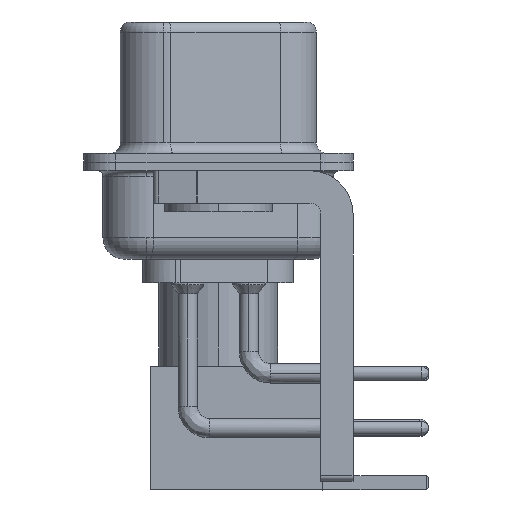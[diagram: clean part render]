
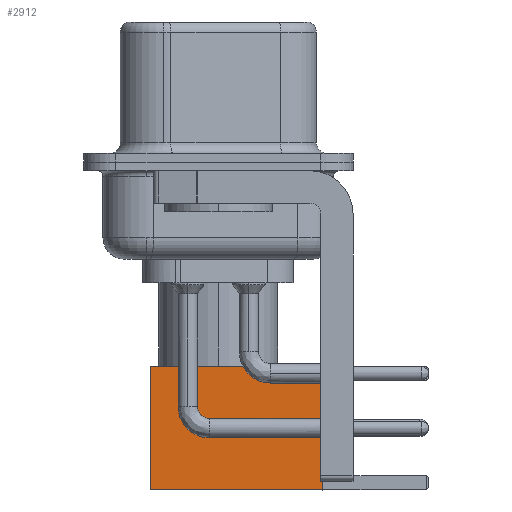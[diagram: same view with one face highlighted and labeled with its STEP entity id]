
A CAD part, left-side view. The second image highlights one B-rep face of the part: STEP entity #2912.
In plain terms, the highlighted face is planar.
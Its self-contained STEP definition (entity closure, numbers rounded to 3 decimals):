
#334 = AXIS2_PLACEMENT_3D ( 'NONE', #9749, #5751, #1366 ) ;
#508 = VECTOR ( 'NONE', #3335, 1000. ) ;
#1143 = LINE ( 'NONE', #26231, #508 ) ;
#1366 = DIRECTION ( 'NONE',  ( 0., 0., 1. ) ) ;
#2645 = EDGE_LOOP ( 'NONE', ( #25051, #9205, #20973, #20475 ) ) ;
#2912 = ADVANCED_FACE ( 'NONE', ( #20149 ), #16172, .T. ) ;
#3005 = VECTOR ( 'NONE', #14137, 1000. ) ;
#3335 = DIRECTION ( 'NONE',  ( 0., 0., -1. ) ) ;
#4708 = CARTESIAN_POINT ( 'NONE',  ( -2.875, 2.875, 0. ) ) ;
#5092 = VERTEX_POINT ( 'NONE', #23687 ) ;
#5507 = VERTEX_POINT ( 'NONE', #12978 ) ;
#5751 = DIRECTION ( 'NONE',  ( 0., 1., 0. ) ) ;
#6274 = VECTOR ( 'NONE', #23021, 1000. ) ;
#8131 = VERTEX_POINT ( 'NONE', #4708 ) ;
#9205 = ORIENTED_EDGE ( 'NONE', *, *, #24511, .T. ) ;
#9615 = EDGE_CURVE ( 'NONE', #5507, #12954, #1143, .T. ) ;
#9749 = CARTESIAN_POINT ( 'NONE',  ( 2.875, 2.875, 0. ) ) ;
#9893 = CARTESIAN_POINT ( 'NONE',  ( -2.875, 2.875, 0. ) ) ;
#12954 = VERTEX_POINT ( 'NONE', #23601 ) ;
#12978 = CARTESIAN_POINT ( 'NONE',  ( 2.875, 2.875, 8. ) ) ;
#14137 = DIRECTION ( 'NONE',  ( 0., 0., -1. ) ) ;
#14679 = LINE ( 'NONE', #20717, #6274 ) ;
#14908 = VECTOR ( 'NONE', #16520, 1000. ) ;
#15547 = EDGE_CURVE ( 'NONE', #5092, #8131, #18251, .T. ) ;
#16172 = PLANE ( 'NONE',  #334 ) ;
#16520 = DIRECTION ( 'NONE',  ( -1., 0., 0. ) ) ;
#18251 = LINE ( 'NONE', #9893, #3005 ) ;
#18891 = EDGE_CURVE ( 'NONE', #5507, #5092, #22675, .T. ) ;
#20149 = FACE_OUTER_BOUND ( 'NONE', #2645, .T. ) ;
#20475 = ORIENTED_EDGE ( 'NONE', *, *, #18891, .F. ) ;
#20717 = CARTESIAN_POINT ( 'NONE',  ( 0., 2.875, 0. ) ) ;
#20973 = ORIENTED_EDGE ( 'NONE', *, *, #15547, .F. ) ;
#22675 = LINE ( 'NONE', #25006, #14908 ) ;
#23021 = DIRECTION ( 'NONE',  ( -1., 0., 0. ) ) ;
#23601 = CARTESIAN_POINT ( 'NONE',  ( 2.875, 2.875, 0. ) ) ;
#23687 = CARTESIAN_POINT ( 'NONE',  ( -2.875, 2.875, 8. ) ) ;
#24511 = EDGE_CURVE ( 'NONE', #12954, #8131, #14679, .T. ) ;
#25006 = CARTESIAN_POINT ( 'NONE',  ( 0., 2.875, 8. ) ) ;
#25051 = ORIENTED_EDGE ( 'NONE', *, *, #9615, .T. ) ;
#26231 = CARTESIAN_POINT ( 'NONE',  ( 2.875, 2.875, 0. ) ) ;
